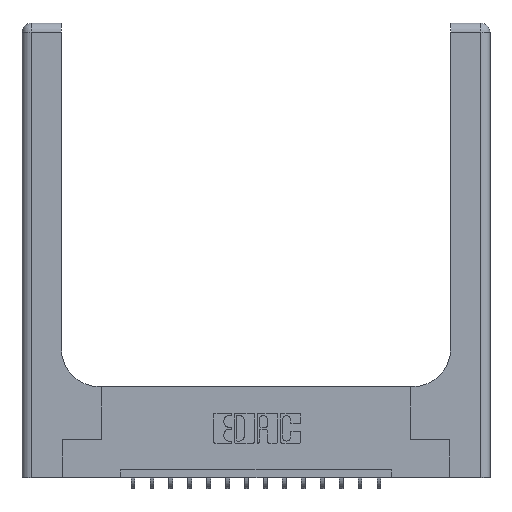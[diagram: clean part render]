
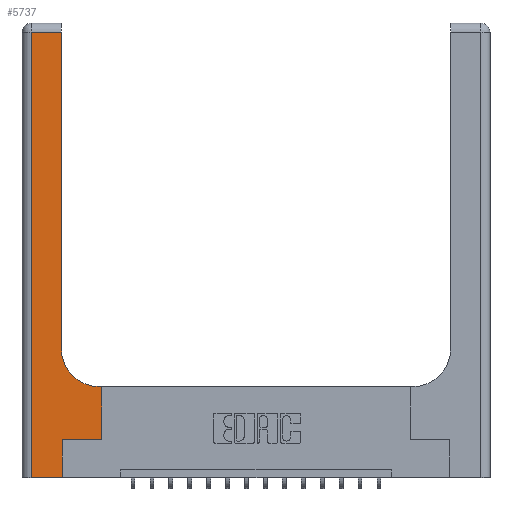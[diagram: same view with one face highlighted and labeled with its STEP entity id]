
A CAD part, top view. The second image highlights one B-rep face of the part: STEP entity #5737.
In plain terms, the highlighted planar face has unit normal (0, 0, 1).
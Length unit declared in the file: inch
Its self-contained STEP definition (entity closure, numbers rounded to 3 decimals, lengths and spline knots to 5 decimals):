
#163 = AXIS2_PLACEMENT_3D ( 'NONE', #3997, #13727, #10964 ) ;
#364 = VECTOR ( 'NONE', #16492, 39.37008 ) ;
#461 = CARTESIAN_POINT ( 'NONE',  ( 0.26, 0.85, 0.37 ) ) ;
#756 = CARTESIAN_POINT ( 'NONE',  ( 0.265, 0.25, 0.37 ) ) ;
#1303 = DIRECTION ( 'NONE',  ( 0., 1., 0. ) ) ;
#1509 = EDGE_CURVE ( 'NONE', #16925, #6244, #3392, .T. ) ;
#1598 = EDGE_LOOP ( 'NONE', ( #17089, #1815, #8620, #1730, #15961, #14972, #5245, #5906, #8903 ) ) ;
#1624 = CIRCLE ( 'NONE', #163, 0.25 ) ;
#1730 = ORIENTED_EDGE ( 'NONE', *, *, #4343, .T. ) ;
#1815 = ORIENTED_EDGE ( 'NONE', *, *, #1509, .T. ) ;
#1977 = DIRECTION ( 'NONE',  ( -1., 0., 0. ) ) ;
#2138 = CARTESIAN_POINT ( 'NONE',  ( 0.528, 0.25, 0.37 ) ) ;
#2151 = VECTOR ( 'NONE', #1303, 39.37008 ) ;
#2870 = VERTEX_POINT ( 'NONE', #17296 ) ;
#3146 = VECTOR ( 'NONE', #17105, 39.37008 ) ;
#3392 = LINE ( 'NONE', #4856, #4072 ) ;
#3512 = CARTESIAN_POINT ( 'NONE',  ( 0.528, 0.25, 0.37 ) ) ;
#3997 = CARTESIAN_POINT ( 'NONE',  ( 0.51, 0.85, 0.37 ) ) ;
#4072 = VECTOR ( 'NONE', #17270, 39.37008 ) ;
#4120 = CARTESIAN_POINT ( 'NONE',  ( 0.26, 3., 0.37 ) ) ;
#4157 = VERTEX_POINT ( 'NONE', #3512 ) ;
#4188 = CARTESIAN_POINT ( 'NONE',  ( 0.528, 0.6, 0.37 ) ) ;
#4343 = EDGE_CURVE ( 'NONE', #10196, #4347, #8640, .T. ) ;
#4347 = VERTEX_POINT ( 'NONE', #4519 ) ;
#4519 = CARTESIAN_POINT ( 'NONE',  ( 0.265, 0., 0.37 ) ) ;
#4856 = CARTESIAN_POINT ( 'NONE',  ( 0., 2.94, 0.37 ) ) ;
#4912 = LINE ( 'NONE', #11692, #6779 ) ;
#4980 = LINE ( 'NONE', #13249, #11373 ) ;
#5223 = EDGE_CURVE ( 'NONE', #4347, #11836, #4980, .T. ) ;
#5245 = ORIENTED_EDGE ( 'NONE', *, *, #8127, .T. ) ;
#5737 = ADVANCED_FACE ( 'NONE', ( #13042 ), #16080, .F. ) ;
#5906 = ORIENTED_EDGE ( 'NONE', *, *, #8881, .T. ) ;
#6244 = VERTEX_POINT ( 'NONE', #16327 ) ;
#6779 = VECTOR ( 'NONE', #1977, 39.37008 ) ;
#7614 = DIRECTION ( 'NONE',  ( 0., 0., -1. ) ) ;
#7894 = EDGE_CURVE ( 'NONE', #11836, #4157, #15924, .T. ) ;
#8127 = EDGE_CURVE ( 'NONE', #4157, #15284, #14709, .T. ) ;
#8620 = ORIENTED_EDGE ( 'NONE', *, *, #8939, .T. ) ;
#8640 = LINE ( 'NONE', #14243, #3146 ) ;
#8881 = EDGE_CURVE ( 'NONE', #15284, #2870, #4912, .T. ) ;
#8903 = ORIENTED_EDGE ( 'NONE', *, *, #14860, .T. ) ;
#8931 = DIRECTION ( 'NONE',  ( 1., 0., 0. ) ) ;
#8939 = EDGE_CURVE ( 'NONE', #6244, #10196, #12256, .T. ) ;
#9087 = CARTESIAN_POINT ( 'NONE',  ( 0., 3., 0.37 ) ) ;
#10177 = DIRECTION ( 'NONE',  ( -1., 0., 0. ) ) ;
#10196 = VERTEX_POINT ( 'NONE', #14314 ) ;
#10904 = LINE ( 'NONE', #4120, #2151 ) ;
#10964 = DIRECTION ( 'NONE',  ( 1., 0., 0. ) ) ;
#11373 = VECTOR ( 'NONE', #13154, 39.37008 ) ;
#11692 = CARTESIAN_POINT ( 'NONE',  ( 0.26, 0.6, 0.37 ) ) ;
#11756 = CARTESIAN_POINT ( 'NONE',  ( 0.26, 2.94, 0.37 ) ) ;
#11836 = VERTEX_POINT ( 'NONE', #756 ) ;
#11974 = AXIS2_PLACEMENT_3D ( 'NONE', #9087, #7614, #10177 ) ;
#12256 = LINE ( 'NONE', #17709, #364 ) ;
#12946 = EDGE_CURVE ( 'NONE', #17549, #16925, #10904, .T. ) ;
#13042 = FACE_OUTER_BOUND ( 'NONE', #1598, .T. ) ;
#13154 = DIRECTION ( 'NONE',  ( 0., 1., 0. ) ) ;
#13249 = CARTESIAN_POINT ( 'NONE',  ( 0.265, 0., 0.37 ) ) ;
#13344 = DIRECTION ( 'NONE',  ( 0., 1., 0. ) ) ;
#13727 = DIRECTION ( 'NONE',  ( 0., 0., -1. ) ) ;
#14243 = CARTESIAN_POINT ( 'NONE',  ( 0., 0., 0.37 ) ) ;
#14314 = CARTESIAN_POINT ( 'NONE',  ( 0.06, 0., 0.37 ) ) ;
#14709 = LINE ( 'NONE', #2138, #17647 ) ;
#14860 = EDGE_CURVE ( 'NONE', #2870, #17549, #1624, .T. ) ;
#14971 = VECTOR ( 'NONE', #8931, 39.37008 ) ;
#14972 = ORIENTED_EDGE ( 'NONE', *, *, #7894, .T. ) ;
#15284 = VERTEX_POINT ( 'NONE', #4188 ) ;
#15924 = LINE ( 'NONE', #17406, #14971 ) ;
#15961 = ORIENTED_EDGE ( 'NONE', *, *, #5223, .T. ) ;
#16080 = PLANE ( 'NONE',  #11974 ) ;
#16327 = CARTESIAN_POINT ( 'NONE',  ( 0.06, 2.94, 0.37 ) ) ;
#16492 = DIRECTION ( 'NONE',  ( 0., -1., 0. ) ) ;
#16925 = VERTEX_POINT ( 'NONE', #11756 ) ;
#17089 = ORIENTED_EDGE ( 'NONE', *, *, #12946, .T. ) ;
#17105 = DIRECTION ( 'NONE',  ( 1., 0., 0. ) ) ;
#17270 = DIRECTION ( 'NONE',  ( -1., 0., 0. ) ) ;
#17296 = CARTESIAN_POINT ( 'NONE',  ( 0.51, 0.6, 0.37 ) ) ;
#17406 = CARTESIAN_POINT ( 'NONE',  ( 0.265, 0.25, 0.37 ) ) ;
#17549 = VERTEX_POINT ( 'NONE', #461 ) ;
#17647 = VECTOR ( 'NONE', #13344, 39.37008 ) ;
#17709 = CARTESIAN_POINT ( 'NONE',  ( 0.06, 3., 0.37 ) ) ;
